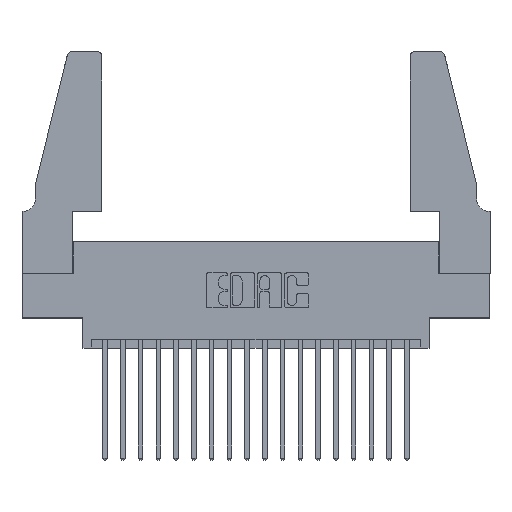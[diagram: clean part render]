
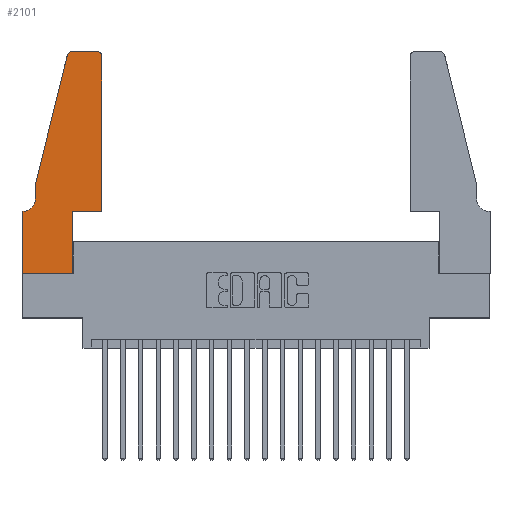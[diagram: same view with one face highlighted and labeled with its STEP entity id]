
A CAD part, top view. The second image highlights one B-rep face of the part: STEP entity #2101.
In plain terms, the highlighted planar face has unit normal (0, 0, 1).
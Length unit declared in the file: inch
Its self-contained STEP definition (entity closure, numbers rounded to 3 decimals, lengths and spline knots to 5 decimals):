
#512 = LINE ( 'NONE', #6947, #4662 ) ;
#724 = EDGE_CURVE ( 'NONE', #7840, #1010, #16105, .T. ) ;
#829 = VERTEX_POINT ( 'NONE', #6617 ) ;
#896 = DIRECTION ( 'NONE',  ( -1., 0., 0. ) ) ;
#1010 = VERTEX_POINT ( 'NONE', #2606 ) ;
#1191 = LINE ( 'NONE', #11623, #4828 ) ;
#1290 = CARTESIAN_POINT ( 'NONE',  ( 0.284, 1.22, 0.37 ) ) ;
#1320 = CARTESIAN_POINT ( 'NONE',  ( 0., 0., 0.37 ) ) ;
#1363 = ORIENTED_EDGE ( 'NONE', *, *, #12583, .T. ) ;
#1581 = CARTESIAN_POINT ( 'NONE',  ( 0.0055, 0.42, 0.37 ) ) ;
#1828 = CARTESIAN_POINT ( 'NONE',  ( 0.4205, 1.22, 0.37 ) ) ;
#1924 = CIRCLE ( 'NONE', #13546, 0.03 ) ;
#2101 = ADVANCED_FACE ( 'NONE', ( #12799 ), #12546, .T. ) ;
#2546 = CARTESIAN_POINT ( 'NONE',  ( 0., 0.35, 0.37 ) ) ;
#2606 = CARTESIAN_POINT ( 'NONE',  ( 0.0755, 0.42, 0.37 ) ) ;
#2764 = ORIENTED_EDGE ( 'NONE', *, *, #10947, .T. ) ;
#2873 = DIRECTION ( 'NONE',  ( 1., 0., 0. ) ) ;
#3064 = ORIENTED_EDGE ( 'NONE', *, *, #12403, .T. ) ;
#3162 = DIRECTION ( 'NONE',  ( -1., 0., 0. ) ) ;
#3401 = DIRECTION ( 'NONE',  ( 1., 0., 0. ) ) ;
#4149 = CIRCLE ( 'NONE', #9987, 0.07 ) ;
#4421 = EDGE_CURVE ( 'NONE', #1010, #4448, #4149, .T. ) ;
#4448 = VERTEX_POINT ( 'NONE', #7825 ) ;
#4622 = CARTESIAN_POINT ( 'NONE',  ( 0., 0., 0.37 ) ) ;
#4662 = VECTOR ( 'NONE', #8486, 39.37008 ) ;
#4828 = VECTOR ( 'NONE', #896, 39.37008 ) ;
#4861 = VERTEX_POINT ( 'NONE', #2546 ) ;
#5886 = CARTESIAN_POINT ( 'NONE',  ( 0.2865, 0.35, 0.37 ) ) ;
#6044 = ORIENTED_EDGE ( 'NONE', *, *, #9155, .T. ) ;
#6207 = DIRECTION ( 'NONE',  ( -0.239, -0.971, 0. ) ) ;
#6617 = CARTESIAN_POINT ( 'NONE',  ( 0.2865, 0.35, 0.37 ) ) ;
#6642 = LINE ( 'NONE', #9851, #14187 ) ;
#6947 = CARTESIAN_POINT ( 'NONE',  ( 0.0755, 0.35, 0.37 ) ) ;
#7448 = LINE ( 'NONE', #4622, #15890 ) ;
#7571 = AXIS2_PLACEMENT_3D ( 'NONE', #15204, #19308, #19478 ) ;
#7825 = CARTESIAN_POINT ( 'NONE',  ( 0.0055, 0.35, 0.37 ) ) ;
#7840 = VERTEX_POINT ( 'NONE', #18907 ) ;
#7909 = ORIENTED_EDGE ( 'NONE', *, *, #17798, .T. ) ;
#8486 = DIRECTION ( 'NONE',  ( -1., 0., 0. ) ) ;
#8550 = ORIENTED_EDGE ( 'NONE', *, *, #18930, .T. ) ;
#8571 = VECTOR ( 'NONE', #19119, 39.37008 ) ;
#8665 = VECTOR ( 'NONE', #16553, 39.37008 ) ;
#9037 = LINE ( 'NONE', #14692, #8571 ) ;
#9155 = EDGE_CURVE ( 'NONE', #9529, #15703, #9037, .T. ) ;
#9261 = EDGE_CURVE ( 'NONE', #10247, #829, #14175, .T. ) ;
#9498 = CARTESIAN_POINT ( 'NONE',  ( 0.4505, 0.35, 0.37 ) ) ;
#9525 = VERTEX_POINT ( 'NONE', #14008 ) ;
#9529 = VERTEX_POINT ( 'NONE', #9498 ) ;
#9851 = CARTESIAN_POINT ( 'NONE',  ( 0.4505, 0.35, 0.37 ) ) ;
#9987 = AXIS2_PLACEMENT_3D ( 'NONE', #1581, #12300, #3162 ) ;
#10247 = VERTEX_POINT ( 'NONE', #12415 ) ;
#10408 = AXIS2_PLACEMENT_3D ( 'NONE', #1828, #12522, #3401 ) ;
#10947 = EDGE_CURVE ( 'NONE', #15703, #15434, #18812, .T. ) ;
#11623 = CARTESIAN_POINT ( 'NONE',  ( 0.2605, 1.25, 0.37 ) ) ;
#12014 = DIRECTION ( 'NONE',  ( 0., 0., 1. ) ) ;
#12131 = VECTOR ( 'NONE', #15917, 39.37008 ) ;
#12142 = CARTESIAN_POINT ( 'NONE',  ( 0., 0., 0.37 ) ) ;
#12300 = DIRECTION ( 'NONE',  ( 0., 0., -1. ) ) ;
#12403 = EDGE_CURVE ( 'NONE', #15434, #9525, #1191, .T. ) ;
#12415 = CARTESIAN_POINT ( 'NONE',  ( 0.2865, 0., 0.37 ) ) ;
#12522 = DIRECTION ( 'NONE',  ( 0., 0., 1. ) ) ;
#12546 = PLANE ( 'NONE',  #7571 ) ;
#12583 = EDGE_CURVE ( 'NONE', #9525, #12703, #1924, .T. ) ;
#12647 = VERTEX_POINT ( 'NONE', #12142 ) ;
#12650 = LINE ( 'NONE', #1320, #8665 ) ;
#12703 = VERTEX_POINT ( 'NONE', #18189 ) ;
#12799 = FACE_OUTER_BOUND ( 'NONE', #15164, .T. ) ;
#13392 = LINE ( 'NONE', #13737, #16927 ) ;
#13397 = CARTESIAN_POINT ( 'NONE',  ( 0.4205, 1.25, 0.37 ) ) ;
#13546 = AXIS2_PLACEMENT_3D ( 'NONE', #1290, #12014, #2873 ) ;
#13737 = CARTESIAN_POINT ( 'NONE',  ( 0.0755, 0.5, 0.37 ) ) ;
#13894 = EDGE_CURVE ( 'NONE', #4448, #4861, #512, .T. ) ;
#14008 = CARTESIAN_POINT ( 'NONE',  ( 0.284, 1.25, 0.37 ) ) ;
#14175 = LINE ( 'NONE', #5886, #18134 ) ;
#14187 = VECTOR ( 'NONE', #17364, 39.37008 ) ;
#14692 = CARTESIAN_POINT ( 'NONE',  ( 0.4505, 0.35, 0.37 ) ) ;
#14923 = EDGE_CURVE ( 'NONE', #12703, #7840, #13392, .T. ) ;
#15164 = EDGE_LOOP ( 'NONE', ( #3064, #1363, #16501, #15931, #17554, #15472, #17289, #7909, #15968, #8550, #6044, #2764 ) ) ;
#15204 = CARTESIAN_POINT ( 'NONE',  ( 0., 0.35, 0.37 ) ) ;
#15434 = VERTEX_POINT ( 'NONE', #13397 ) ;
#15472 = ORIENTED_EDGE ( 'NONE', *, *, #13894, .T. ) ;
#15703 = VERTEX_POINT ( 'NONE', #18420 ) ;
#15890 = VECTOR ( 'NONE', #16726, 39.37008 ) ;
#15917 = DIRECTION ( 'NONE',  ( 0., -1., 0. ) ) ;
#15931 = ORIENTED_EDGE ( 'NONE', *, *, #724, .T. ) ;
#15968 = ORIENTED_EDGE ( 'NONE', *, *, #9261, .T. ) ;
#16105 = LINE ( 'NONE', #19248, #12131 ) ;
#16449 = DIRECTION ( 'NONE',  ( 0., 1., 0. ) ) ;
#16501 = ORIENTED_EDGE ( 'NONE', *, *, #14923, .T. ) ;
#16553 = DIRECTION ( 'NONE',  ( 0., -1., 0. ) ) ;
#16726 = DIRECTION ( 'NONE',  ( 1., 0., 0. ) ) ;
#16927 = VECTOR ( 'NONE', #6207, 39.37008 ) ;
#17148 = EDGE_CURVE ( 'NONE', #4861, #12647, #12650, .T. ) ;
#17289 = ORIENTED_EDGE ( 'NONE', *, *, #17148, .T. ) ;
#17364 = DIRECTION ( 'NONE',  ( 1., 0., 0. ) ) ;
#17554 = ORIENTED_EDGE ( 'NONE', *, *, #4421, .T. ) ;
#17798 = EDGE_CURVE ( 'NONE', #12647, #10247, #7448, .T. ) ;
#18134 = VECTOR ( 'NONE', #16449, 39.37008 ) ;
#18189 = CARTESIAN_POINT ( 'NONE',  ( 0.25487, 1.22718, 0.37 ) ) ;
#18420 = CARTESIAN_POINT ( 'NONE',  ( 0.4505, 1.22, 0.37 ) ) ;
#18812 = CIRCLE ( 'NONE', #10408, 0.03 ) ;
#18907 = CARTESIAN_POINT ( 'NONE',  ( 0.0755, 0.5, 0.37 ) ) ;
#18930 = EDGE_CURVE ( 'NONE', #829, #9529, #6642, .T. ) ;
#19119 = DIRECTION ( 'NONE',  ( 0., 1., 0. ) ) ;
#19248 = CARTESIAN_POINT ( 'NONE',  ( 0.0755, 0.5, 0.37 ) ) ;
#19308 = DIRECTION ( 'NONE',  ( 0., 0., 1. ) ) ;
#19478 = DIRECTION ( 'NONE',  ( 1., 0., 0. ) ) ;
